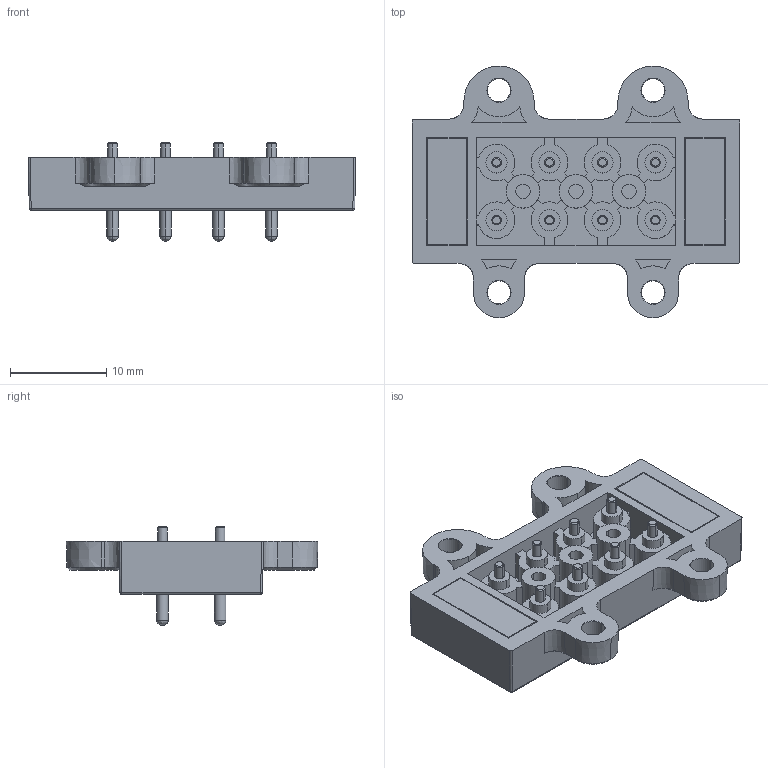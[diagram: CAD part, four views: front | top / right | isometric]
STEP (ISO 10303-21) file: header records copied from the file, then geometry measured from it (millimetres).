
FILE_DESCRIPTION (( 'STEP AP203' ), '1' );
FILE_NAME ('685A0811221113E.STEP', '2023-03-01T12:49:46', ( 'Magnum' ), ( '' ), 'SwSTEP 2.0', 'SolidWorks 2020', '' );
FILE_SCHEMA (( 'CONFIG_CONTROL_DESIGN' ));
Length unit declared in the file: millimetre
Products named in the file (1): 685A0811221113E
Bounding box: 34 x 26.15 x 10.2 mm (x, y, z)
Volume: 2580.1 mm3; surface area: 3469.5 mm2
Topology: 9 solids, 11 shells, 412 faces, 991 edges, 639 vertices
Faces by surface type: plane 208, cylinder 132, cone 44, bspline 16, torus 8, sphere 4
Entity records: 12534 total; most frequent: CARTESIAN_POINT 2580, DIRECTION 2157, ORIENTED_EDGE 1982, EDGE_CURVE 991, AXIS2_PLACEMENT_3D 788, VERTEX_POINT 639, VECTOR 581, LINE 581
